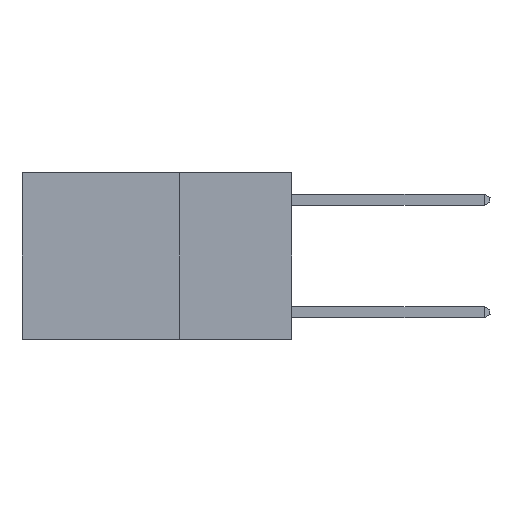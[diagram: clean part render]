
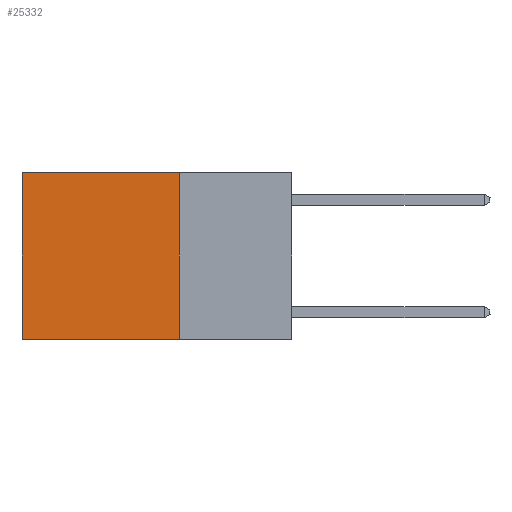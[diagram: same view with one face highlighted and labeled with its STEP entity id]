
A CAD part, left-side view. The second image highlights one B-rep face of the part: STEP entity #25332.
In plain terms, the highlighted planar face has unit normal (-1, 0, 0).
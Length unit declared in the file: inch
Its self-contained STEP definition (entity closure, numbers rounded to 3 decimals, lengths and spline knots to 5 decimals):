
#560 = PLANE ( 'NONE',  #24471 ) ;
#902 = VERTEX_POINT ( 'NONE', #7695 ) ;
#2450 = LINE ( 'NONE', #7140, #24169 ) ;
#3462 = EDGE_CURVE ( 'NONE', #18066, #9865, #2450, .T. ) ;
#3648 = EDGE_CURVE ( 'NONE', #18066, #9292, #6468, .T. ) ;
#3703 = EDGE_CURVE ( 'NONE', #9292, #902, #23167, .T. ) ;
#4750 = DIRECTION ( 'NONE',  ( 0., 0., -1. ) ) ;
#4937 = LINE ( 'NONE', #13058, #20258 ) ;
#5223 = VECTOR ( 'NONE', #20783, 39.37008 ) ;
#6468 = LINE ( 'NONE', #22756, #5223 ) ;
#7140 = CARTESIAN_POINT ( 'NONE',  ( 0.2625, 0.25, 0. ) ) ;
#7695 = CARTESIAN_POINT ( 'NONE',  ( 0.2625, 0.6, -0.37 ) ) ;
#8154 = ORIENTED_EDGE ( 'NONE', *, *, #3703, .T. ) ;
#8530 = ORIENTED_EDGE ( 'NONE', *, *, #3462, .F. ) ;
#9292 = VERTEX_POINT ( 'NONE', #11380 ) ;
#9865 = VERTEX_POINT ( 'NONE', #23992 ) ;
#10011 = CARTESIAN_POINT ( 'NONE',  ( 0.2625, 0.25, 0. ) ) ;
#10172 = FACE_OUTER_BOUND ( 'NONE', #23415, .T. ) ;
#11380 = CARTESIAN_POINT ( 'NONE',  ( 0.2625, 0.6, 0. ) ) ;
#13058 = CARTESIAN_POINT ( 'NONE',  ( 0.2625, 0.25, -0.37 ) ) ;
#13849 = ORIENTED_EDGE ( 'NONE', *, *, #3648, .T. ) ;
#14225 = ORIENTED_EDGE ( 'NONE', *, *, #25890, .F. ) ;
#18066 = VERTEX_POINT ( 'NONE', #10011 ) ;
#20036 = VECTOR ( 'NONE', #22753, 39.37008 ) ;
#20258 = VECTOR ( 'NONE', #21080, 39.37008 ) ;
#20732 = DIRECTION ( 'NONE',  ( 1., 0., 0. ) ) ;
#20783 = DIRECTION ( 'NONE',  ( 0., 1., 0. ) ) ;
#21080 = DIRECTION ( 'NONE',  ( 0., 1., 0. ) ) ;
#21183 = CARTESIAN_POINT ( 'NONE',  ( 0.2625, 0.6, 0. ) ) ;
#22753 = DIRECTION ( 'NONE',  ( 0., 0., -1. ) ) ;
#22756 = CARTESIAN_POINT ( 'NONE',  ( 0.2625, 0.25, 0. ) ) ;
#23167 = LINE ( 'NONE', #21183, #20036 ) ;
#23415 = EDGE_LOOP ( 'NONE', ( #8154, #14225, #8530, #13849 ) ) ;
#23992 = CARTESIAN_POINT ( 'NONE',  ( 0.2625, 0.25, -0.37 ) ) ;
#24169 = VECTOR ( 'NONE', #4750, 39.37008 ) ;
#24447 = CARTESIAN_POINT ( 'NONE',  ( 0.2625, 0.25, 0. ) ) ;
#24471 = AXIS2_PLACEMENT_3D ( 'NONE', #24447, #20732, #24587 ) ;
#24587 = DIRECTION ( 'NONE',  ( 0., 0., -1. ) ) ;
#25332 = ADVANCED_FACE ( 'NONE', ( #10172 ), #560, .F. ) ;
#25890 = EDGE_CURVE ( 'NONE', #9865, #902, #4937, .T. ) ;
